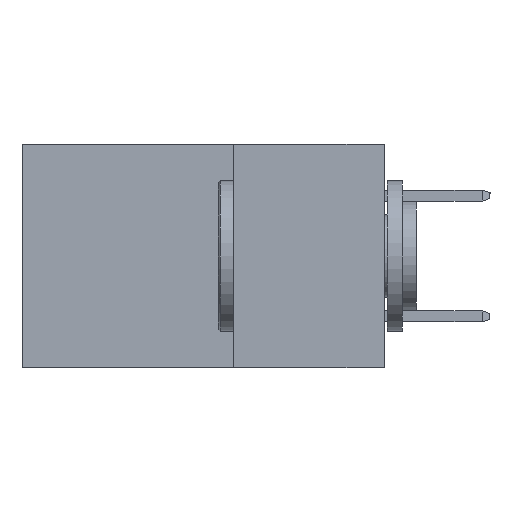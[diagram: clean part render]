
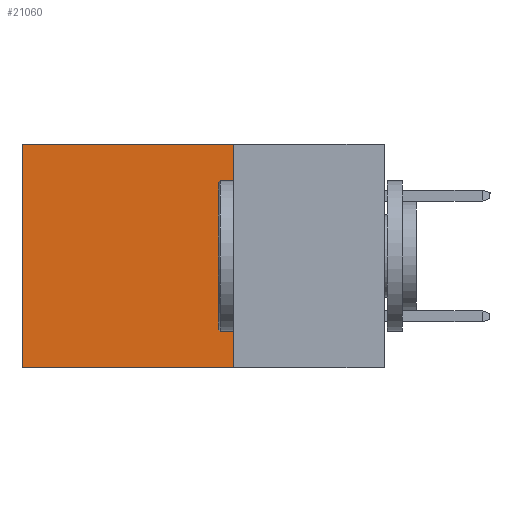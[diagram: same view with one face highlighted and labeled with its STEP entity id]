
A CAD part, left-side view. The second image highlights one B-rep face of the part: STEP entity #21060.
In plain terms, the highlighted planar face has unit normal (-1, 0, 0).
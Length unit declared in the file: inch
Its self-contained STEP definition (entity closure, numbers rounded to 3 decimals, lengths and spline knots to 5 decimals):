
#43 = LINE ( 'NONE', #8016, #13323 ) ;
#194 = CARTESIAN_POINT ( 'NONE',  ( 0.2615, 0.25, -0.37 ) ) ;
#384 = VERTEX_POINT ( 'NONE', #6654 ) ;
#602 = CARTESIAN_POINT ( 'NONE',  ( 0.2615, 0.25, 0. ) ) ;
#631 = DIRECTION ( 'NONE',  ( 0., 1., 0. ) ) ;
#646 = AXIS2_PLACEMENT_3D ( 'NONE', #2765, #13826, #23810 ) ;
#715 = EDGE_CURVE ( 'NONE', #16453, #23006, #743, .T. ) ;
#743 = LINE ( 'NONE', #4363, #12361 ) ;
#2765 = CARTESIAN_POINT ( 'NONE',  ( 0.2615, 0.25, -0.37 ) ) ;
#4283 = EDGE_CURVE ( 'NONE', #23006, #384, #23452, .T. ) ;
#4363 = CARTESIAN_POINT ( 'NONE',  ( 0.2615, 0.25, 0. ) ) ;
#5806 = EDGE_LOOP ( 'NONE', ( #20912, #11879, #16203, #6901 ) ) ;
#6654 = CARTESIAN_POINT ( 'NONE',  ( 0.2615, 0.6, -0.37 ) ) ;
#6656 = EDGE_CURVE ( 'NONE', #14268, #384, #7983, .T. ) ;
#6901 = ORIENTED_EDGE ( 'NONE', *, *, #715, .T. ) ;
#7882 = EDGE_CURVE ( 'NONE', #16453, #14268, #43, .T. ) ;
#7983 = LINE ( 'NONE', #12021, #13211 ) ;
#8016 = CARTESIAN_POINT ( 'NONE',  ( 0.2615, 0.25, -0.37 ) ) ;
#11879 = ORIENTED_EDGE ( 'NONE', *, *, #6656, .F. ) ;
#12021 = CARTESIAN_POINT ( 'NONE',  ( 0.2615, 0.25, -0.37 ) ) ;
#12361 = VECTOR ( 'NONE', #16015, 39.37008 ) ;
#13211 = VECTOR ( 'NONE', #631, 39.37008 ) ;
#13323 = VECTOR ( 'NONE', #23076, 39.37008 ) ;
#13699 = FACE_OUTER_BOUND ( 'NONE', #5806, .T. ) ;
#13826 = DIRECTION ( 'NONE',  ( 1., 0., 0. ) ) ;
#14198 = CARTESIAN_POINT ( 'NONE',  ( 0.2615, 0.6, -0.37 ) ) ;
#14268 = VERTEX_POINT ( 'NONE', #194 ) ;
#16015 = DIRECTION ( 'NONE',  ( 0., 1., 0. ) ) ;
#16203 = ORIENTED_EDGE ( 'NONE', *, *, #7882, .F. ) ;
#16453 = VERTEX_POINT ( 'NONE', #602 ) ;
#17784 = VECTOR ( 'NONE', #21943, 39.37008 ) ;
#17828 = PLANE ( 'NONE',  #646 ) ;
#18734 = CARTESIAN_POINT ( 'NONE',  ( 0.2615, 0.6, 0. ) ) ;
#20912 = ORIENTED_EDGE ( 'NONE', *, *, #4283, .T. ) ;
#21060 = ADVANCED_FACE ( 'NONE', ( #13699 ), #17828, .F. ) ;
#21943 = DIRECTION ( 'NONE',  ( 0., 0., -1. ) ) ;
#23006 = VERTEX_POINT ( 'NONE', #18734 ) ;
#23076 = DIRECTION ( 'NONE',  ( 0., 0., -1. ) ) ;
#23452 = LINE ( 'NONE', #14198, #17784 ) ;
#23810 = DIRECTION ( 'NONE',  ( 0., 0., -1. ) ) ;
